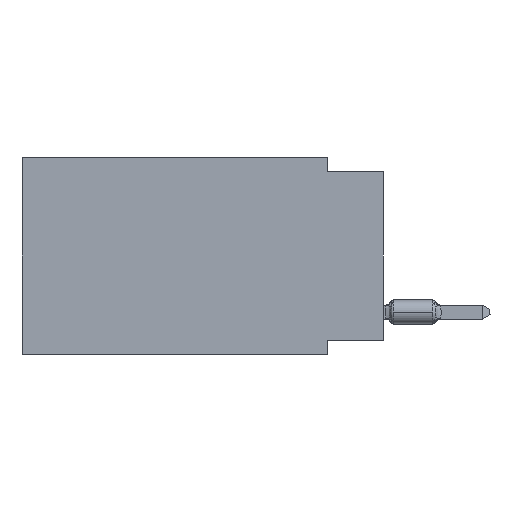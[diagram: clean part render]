
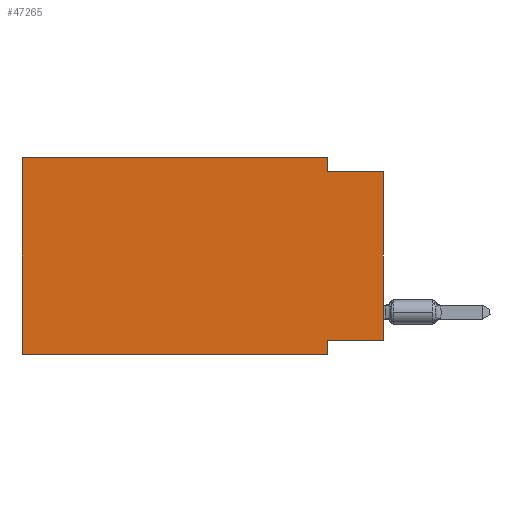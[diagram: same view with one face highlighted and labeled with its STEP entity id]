
A CAD part, left-side view. The second image highlights one B-rep face of the part: STEP entity #47265.
In plain terms, the highlighted planar face has unit normal (-1, 0, 0).
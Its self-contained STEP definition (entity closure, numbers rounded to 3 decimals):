
#894 = EDGE_CURVE ( 'NONE', #49090, #12772, #21537, .T. ) ;
#2646 = LINE ( 'NONE', #35587, #17331 ) ;
#4068 = LINE ( 'NONE', #53129, #31726 ) ;
#4535 = LINE ( 'NONE', #54675, #23875 ) ;
#5562 = CARTESIAN_POINT ( 'NONE',  ( 0., 0., -0.635 ) ) ;
#5925 = DIRECTION ( 'NONE',  ( 0., -1., 0. ) ) ;
#6152 = PLANE ( 'NONE',  #41058 ) ;
#6820 = EDGE_LOOP ( 'NONE', ( #37542, #42848, #46985, #55545, #69698, #68903, #48673, #11283 ) ) ;
#7682 = CARTESIAN_POINT ( 'NONE',  ( 0., 2.54, 0. ) ) ;
#8501 = DIRECTION ( 'NONE',  ( 0., 0., 1. ) ) ;
#8705 = CARTESIAN_POINT ( 'NONE',  ( 0., 2.54, -0.635 ) ) ;
#10574 = EDGE_CURVE ( 'NONE', #16167, #33960, #2646, .T. ) ;
#10743 = CARTESIAN_POINT ( 'NONE',  ( 0., 2.54, -8.89 ) ) ;
#11283 = ORIENTED_EDGE ( 'NONE', *, *, #36960, .F. ) ;
#11969 = DIRECTION ( 'NONE',  ( 0., 0., -1. ) ) ;
#12772 = VERTEX_POINT ( 'NONE', #8705 ) ;
#14785 = DIRECTION ( 'NONE',  ( 0., 0., 1. ) ) ;
#15382 = EDGE_CURVE ( 'NONE', #12772, #33960, #62262, .T. ) ;
#16167 = VERTEX_POINT ( 'NONE', #34204 ) ;
#17331 = VECTOR ( 'NONE', #8501, 1000. ) ;
#18668 = DIRECTION ( 'NONE',  ( 0., 1., 0. ) ) ;
#21225 = VERTEX_POINT ( 'NONE', #41553 ) ;
#21537 = LINE ( 'NONE', #38343, #33677 ) ;
#21873 = CARTESIAN_POINT ( 'NONE',  ( 0., 2.54, -8.255 ) ) ;
#22632 = FACE_OUTER_BOUND ( 'NONE', #6820, .T. ) ;
#23875 = VECTOR ( 'NONE', #14785, 1000. ) ;
#26117 = VECTOR ( 'NONE', #18668, 1000. ) ;
#26921 = VECTOR ( 'NONE', #50126, 1000. ) ;
#27818 = LINE ( 'NONE', #57041, #26921 ) ;
#30732 = VECTOR ( 'NONE', #5925, 1000. ) ;
#31726 = VECTOR ( 'NONE', #64820, 1000. ) ;
#33677 = VECTOR ( 'NONE', #37986, 1000. ) ;
#33960 = VERTEX_POINT ( 'NONE', #47048 ) ;
#34204 = CARTESIAN_POINT ( 'NONE',  ( 0., 0., -8.255 ) ) ;
#34812 = VERTEX_POINT ( 'NONE', #35433 ) ;
#35433 = CARTESIAN_POINT ( 'NONE',  ( 0., 16.383, -8.89 ) ) ;
#35587 = CARTESIAN_POINT ( 'NONE',  ( 0., 0., 0. ) ) ;
#36587 = CARTESIAN_POINT ( 'NONE',  ( 0., 0., -8.255 ) ) ;
#36960 = EDGE_CURVE ( 'NONE', #16167, #57424, #64039, .T. ) ;
#37542 = ORIENTED_EDGE ( 'NONE', *, *, #10574, .T. ) ;
#37770 = EDGE_CURVE ( 'NONE', #34812, #21225, #4535, .T. ) ;
#37986 = DIRECTION ( 'NONE',  ( 0., 0., -1. ) ) ;
#38343 = CARTESIAN_POINT ( 'NONE',  ( 0., 2.54, 0. ) ) ;
#39452 = DIRECTION ( 'NONE',  ( 0., 0., -1. ) ) ;
#41058 = AXIS2_PLACEMENT_3D ( 'NONE', #67624, #44947, #39452 ) ;
#41553 = CARTESIAN_POINT ( 'NONE',  ( 0., 16.383, 0. ) ) ;
#42848 = ORIENTED_EDGE ( 'NONE', *, *, #15382, .F. ) ;
#44316 = EDGE_CURVE ( 'NONE', #21225, #49090, #27818, .T. ) ;
#44947 = DIRECTION ( 'NONE',  ( 1., 0., 0. ) ) ;
#46598 = EDGE_CURVE ( 'NONE', #34812, #61443, #4068, .T. ) ;
#46985 = ORIENTED_EDGE ( 'NONE', *, *, #894, .F. ) ;
#47048 = CARTESIAN_POINT ( 'NONE',  ( 0., 0., -0.635 ) ) ;
#47265 = ADVANCED_FACE ( 'NONE', ( #22632 ), #6152, .F. ) ;
#48673 = ORIENTED_EDGE ( 'NONE', *, *, #59897, .F. ) ;
#49090 = VERTEX_POINT ( 'NONE', #7682 ) ;
#50126 = DIRECTION ( 'NONE',  ( 0., -1., 0. ) ) ;
#51852 = CARTESIAN_POINT ( 'NONE',  ( 0., 2.54, -8.89 ) ) ;
#53129 = CARTESIAN_POINT ( 'NONE',  ( 0., 16.383, -8.89 ) ) ;
#54675 = CARTESIAN_POINT ( 'NONE',  ( 0., 16.383, 0. ) ) ;
#55545 = ORIENTED_EDGE ( 'NONE', *, *, #44316, .F. ) ;
#57041 = CARTESIAN_POINT ( 'NONE',  ( 0., 16.383, 0. ) ) ;
#57424 = VERTEX_POINT ( 'NONE', #21873 ) ;
#59897 = EDGE_CURVE ( 'NONE', #57424, #61443, #67603, .T. ) ;
#61443 = VERTEX_POINT ( 'NONE', #10743 ) ;
#62262 = LINE ( 'NONE', #5562, #30732 ) ;
#64039 = LINE ( 'NONE', #36587, #26117 ) ;
#64820 = DIRECTION ( 'NONE',  ( 0., -1., 0. ) ) ;
#66219 = VECTOR ( 'NONE', #11969, 1000. ) ;
#67603 = LINE ( 'NONE', #51852, #66219 ) ;
#67624 = CARTESIAN_POINT ( 'NONE',  ( 0., 16.383, 0. ) ) ;
#68903 = ORIENTED_EDGE ( 'NONE', *, *, #46598, .T. ) ;
#69698 = ORIENTED_EDGE ( 'NONE', *, *, #37770, .F. ) ;
